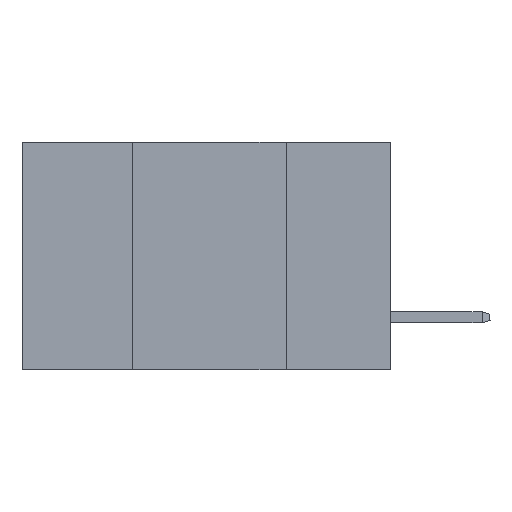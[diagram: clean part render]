
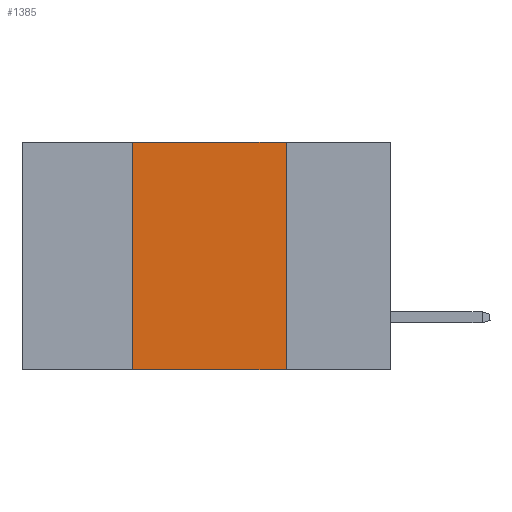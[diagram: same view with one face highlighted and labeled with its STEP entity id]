
A CAD part, left-side view. The second image highlights one B-rep face of the part: STEP entity #1385.
In plain terms, the highlighted planar face has unit normal (-1, 0, 0).
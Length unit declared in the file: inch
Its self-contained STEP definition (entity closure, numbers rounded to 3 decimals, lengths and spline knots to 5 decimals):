
#1385 = ADVANCED_FACE ( 'NONE', ( #9838 ), #10521, .F. ) ;
#1419 = CARTESIAN_POINT ( 'NONE',  ( 0., 0.42, 0. ) ) ;
#1965 = EDGE_LOOP ( 'NONE', ( #13558, #5087, #15459, #9178 ) ) ;
#2106 = LINE ( 'NONE', #12259, #12741 ) ;
#2373 = VECTOR ( 'NONE', #7706, 39.37008 ) ;
#2672 = EDGE_CURVE ( 'NONE', #3904, #5860, #5613, .T. ) ;
#3195 = LINE ( 'NONE', #4163, #13257 ) ;
#3250 = DIRECTION ( 'NONE',  ( 1., 0., 0. ) ) ;
#3411 = EDGE_CURVE ( 'NONE', #4208, #3619, #2106, .T. ) ;
#3517 = CARTESIAN_POINT ( 'NONE',  ( 0., 0.6, 0. ) ) ;
#3619 = VERTEX_POINT ( 'NONE', #6304 ) ;
#3904 = VERTEX_POINT ( 'NONE', #15221 ) ;
#4163 = CARTESIAN_POINT ( 'NONE',  ( 0., 0.17, 0. ) ) ;
#4208 = VERTEX_POINT ( 'NONE', #1419 ) ;
#5003 = EDGE_CURVE ( 'NONE', #3619, #5860, #3195, .T. ) ;
#5087 = ORIENTED_EDGE ( 'NONE', *, *, #3411, .F. ) ;
#5613 = LINE ( 'NONE', #11279, #2373 ) ;
#5657 = DIRECTION ( 'NONE',  ( 0., 0., -1. ) ) ;
#5860 = VERTEX_POINT ( 'NONE', #10398 ) ;
#6062 = LINE ( 'NONE', #14117, #7387 ) ;
#6304 = CARTESIAN_POINT ( 'NONE',  ( 0., 0.17, 0. ) ) ;
#7387 = VECTOR ( 'NONE', #11824, 39.37008 ) ;
#7706 = DIRECTION ( 'NONE',  ( 0., -1., 0. ) ) ;
#9178 = ORIENTED_EDGE ( 'NONE', *, *, #2672, .T. ) ;
#9838 = FACE_OUTER_BOUND ( 'NONE', #1965, .T. ) ;
#10398 = CARTESIAN_POINT ( 'NONE',  ( 0., 0.17, -0.37 ) ) ;
#10521 = PLANE ( 'NONE',  #14124 ) ;
#11279 = CARTESIAN_POINT ( 'NONE',  ( 0., 0.6, -0.37 ) ) ;
#11824 = DIRECTION ( 'NONE',  ( 0., 0., 1. ) ) ;
#12259 = CARTESIAN_POINT ( 'NONE',  ( 0., 0.6, 0. ) ) ;
#12313 = DIRECTION ( 'NONE',  ( 0., 0., -1. ) ) ;
#12741 = VECTOR ( 'NONE', #14515, 39.37008 ) ;
#13059 = EDGE_CURVE ( 'NONE', #3904, #4208, #6062, .T. ) ;
#13257 = VECTOR ( 'NONE', #12313, 39.37008 ) ;
#13558 = ORIENTED_EDGE ( 'NONE', *, *, #5003, .F. ) ;
#14117 = CARTESIAN_POINT ( 'NONE',  ( 0., 0.42, 0. ) ) ;
#14124 = AXIS2_PLACEMENT_3D ( 'NONE', #3517, #3250, #5657 ) ;
#14515 = DIRECTION ( 'NONE',  ( 0., -1., 0. ) ) ;
#15221 = CARTESIAN_POINT ( 'NONE',  ( 0., 0.42, -0.37 ) ) ;
#15459 = ORIENTED_EDGE ( 'NONE', *, *, #13059, .F. ) ;
